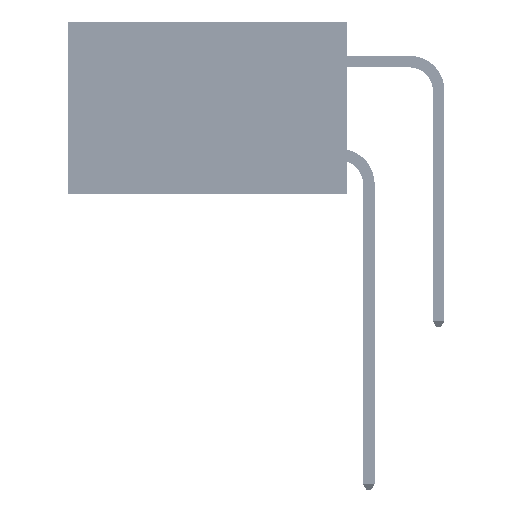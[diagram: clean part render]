
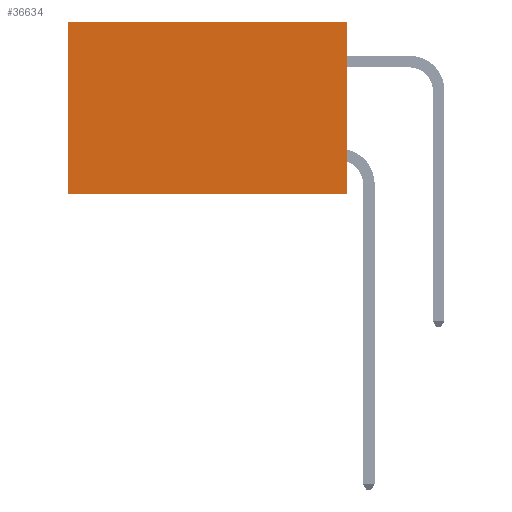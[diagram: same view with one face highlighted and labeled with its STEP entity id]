
A CAD part, left-side view. The second image highlights one B-rep face of the part: STEP entity #36634.
In plain terms, the highlighted planar face has unit normal (-1, 0, 0).
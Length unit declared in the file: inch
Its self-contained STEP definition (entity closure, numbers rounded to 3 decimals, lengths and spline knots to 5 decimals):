
#3758 = CARTESIAN_POINT ( 'NONE',  ( 0.2875, 0., 0. ) ) ;
#4030 = CARTESIAN_POINT ( 'NONE',  ( 0.2875, 0., 0. ) ) ;
#7236 = LINE ( 'NONE', #15524, #10217 ) ;
#8245 = DIRECTION ( 'NONE',  ( 0., 1., 0. ) ) ;
#9016 = CARTESIAN_POINT ( 'NONE',  ( 0.2875, 0., 0. ) ) ;
#9208 = LINE ( 'NONE', #3758, #36029 ) ;
#10217 = VECTOR ( 'NONE', #46197, 39.37008 ) ;
#11928 = VERTEX_POINT ( 'NONE', #4030 ) ;
#12705 = VERTEX_POINT ( 'NONE', #38287 ) ;
#13442 = CARTESIAN_POINT ( 'NONE',  ( 0.2875, 0., 0. ) ) ;
#15524 = CARTESIAN_POINT ( 'NONE',  ( 0.2875, 0.6, 0. ) ) ;
#16992 = DIRECTION ( 'NONE',  ( 0., 0., -1. ) ) ;
#18994 = CARTESIAN_POINT ( 'NONE',  ( 0.2875, 0., -0.37 ) ) ;
#19061 = ORIENTED_EDGE ( 'NONE', *, *, #44967, .T. ) ;
#21291 = EDGE_LOOP ( 'NONE', ( #27734, #38467, #38203, #19061 ) ) ;
#22107 = VERTEX_POINT ( 'NONE', #47885 ) ;
#23515 = AXIS2_PLACEMENT_3D ( 'NONE', #13442, #36319, #44473 ) ;
#23562 = CARTESIAN_POINT ( 'NONE',  ( 0.2875, 0., -0.37 ) ) ;
#25159 = PLANE ( 'NONE',  #23515 ) ;
#27734 = ORIENTED_EDGE ( 'NONE', *, *, #33593, .T. ) ;
#27798 = LINE ( 'NONE', #23562, #28414 ) ;
#27830 = EDGE_CURVE ( 'NONE', #11928, #42679, #35100, .T. ) ;
#28414 = VECTOR ( 'NONE', #8245, 39.37008 ) ;
#29766 = DIRECTION ( 'NONE',  ( 0., 1., 0. ) ) ;
#33593 = EDGE_CURVE ( 'NONE', #12705, #22107, #7236, .T. ) ;
#35100 = LINE ( 'NONE', #9016, #44052 ) ;
#35689 = EDGE_CURVE ( 'NONE', #42679, #22107, #27798, .T. ) ;
#36029 = VECTOR ( 'NONE', #29766, 39.37008 ) ;
#36319 = DIRECTION ( 'NONE',  ( 1., 0., 0. ) ) ;
#36634 = ADVANCED_FACE ( 'NONE', ( #44379 ), #25159, .F. ) ;
#38203 = ORIENTED_EDGE ( 'NONE', *, *, #27830, .F. ) ;
#38287 = CARTESIAN_POINT ( 'NONE',  ( 0.2875, 0.6, 0. ) ) ;
#38467 = ORIENTED_EDGE ( 'NONE', *, *, #35689, .F. ) ;
#42679 = VERTEX_POINT ( 'NONE', #18994 ) ;
#44052 = VECTOR ( 'NONE', #16992, 39.37008 ) ;
#44379 = FACE_OUTER_BOUND ( 'NONE', #21291, .T. ) ;
#44473 = DIRECTION ( 'NONE',  ( 0., 0., -1. ) ) ;
#44967 = EDGE_CURVE ( 'NONE', #11928, #12705, #9208, .T. ) ;
#46197 = DIRECTION ( 'NONE',  ( 0., 0., -1. ) ) ;
#47885 = CARTESIAN_POINT ( 'NONE',  ( 0.2875, 0.6, -0.37 ) ) ;
